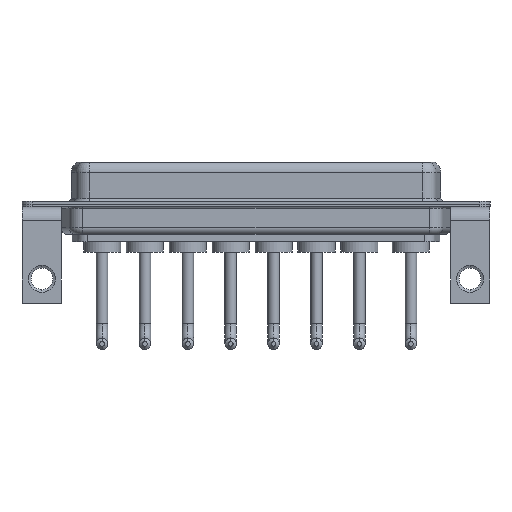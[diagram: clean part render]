
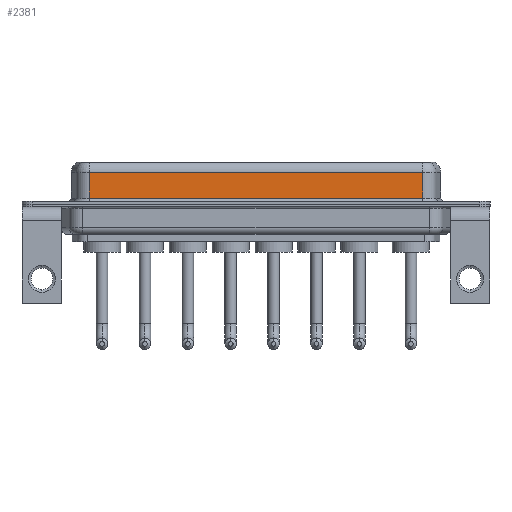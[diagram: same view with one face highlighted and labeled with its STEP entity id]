
A CAD part, front view. The second image highlights one B-rep face of the part: STEP entity #2381.
In plain terms, the highlighted planar face has unit normal (0, -1, 0).
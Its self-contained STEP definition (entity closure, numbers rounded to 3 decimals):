
#185 = VERTEX_POINT ( 'NONE', #13521 ) ;
#1235 = CARTESIAN_POINT ( 'NONE',  ( 56.462, -3.95, 0.9 ) ) ;
#1314 = CARTESIAN_POINT ( 'NONE',  ( 56.462, -3.95, 0.9 ) ) ;
#1459 = ORIENTED_EDGE ( 'NONE', *, *, #13562, .T. ) ;
#1554 = CARTESIAN_POINT ( 'NONE',  ( 7.038, -3.95, 0.9 ) ) ;
#1815 = DIRECTION ( 'NONE',  ( -1., 0., 0. ) ) ;
#2146 = VECTOR ( 'NONE', #1815, 1000. ) ;
#2158 = DIRECTION ( 'NONE',  ( 1., 0., 0. ) ) ;
#2282 = CARTESIAN_POINT ( 'NONE',  ( 56.462, -3.95, 4.65 ) ) ;
#2297 = VECTOR ( 'NONE', #3578, 1000. ) ;
#2381 = ADVANCED_FACE ( 'NONE', ( #13694 ), #3968, .F. ) ;
#2827 = DIRECTION ( 'NONE',  ( 0., 1., 0. ) ) ;
#3151 = EDGE_CURVE ( 'NONE', #6410, #12816, #8992, .T. ) ;
#3353 = CARTESIAN_POINT ( 'NONE',  ( 7.038, -3.95, 4.65 ) ) ;
#3578 = DIRECTION ( 'NONE',  ( 0., 0., -1. ) ) ;
#3968 = PLANE ( 'NONE',  #8597 ) ;
#3984 = EDGE_CURVE ( 'NONE', #13547, #6410, #8546, .T. ) ;
#4740 = DIRECTION ( 'NONE',  ( 0., 0., -1. ) ) ;
#4902 = DIRECTION ( 'NONE',  ( 0., 0., 1. ) ) ;
#5566 = VECTOR ( 'NONE', #4740, 1000. ) ;
#5620 = EDGE_LOOP ( 'NONE', ( #9661, #1459, #6217, #13691 ) ) ;
#6217 = ORIENTED_EDGE ( 'NONE', *, *, #3984, .T. ) ;
#6410 = VERTEX_POINT ( 'NONE', #1554 ) ;
#6791 = LINE ( 'NONE', #10136, #5566 ) ;
#7906 = EDGE_CURVE ( 'NONE', #185, #12816, #6791, .T. ) ;
#8213 = CARTESIAN_POINT ( 'NONE',  ( 56.462, -3.95, 6.4 ) ) ;
#8546 = LINE ( 'NONE', #9109, #2297 ) ;
#8597 = AXIS2_PLACEMENT_3D ( 'NONE', #8213, #2827, #4902 ) ;
#8992 = LINE ( 'NONE', #1235, #11209 ) ;
#9109 = CARTESIAN_POINT ( 'NONE',  ( 7.038, -3.95, 6.4 ) ) ;
#9661 = ORIENTED_EDGE ( 'NONE', *, *, #7906, .F. ) ;
#10136 = CARTESIAN_POINT ( 'NONE',  ( 56.462, -3.95, 6.4 ) ) ;
#11209 = VECTOR ( 'NONE', #2158, 1000. ) ;
#12034 = LINE ( 'NONE', #2282, #2146 ) ;
#12816 = VERTEX_POINT ( 'NONE', #1314 ) ;
#13521 = CARTESIAN_POINT ( 'NONE',  ( 56.462, -3.95, 4.65 ) ) ;
#13547 = VERTEX_POINT ( 'NONE', #3353 ) ;
#13562 = EDGE_CURVE ( 'NONE', #185, #13547, #12034, .T. ) ;
#13691 = ORIENTED_EDGE ( 'NONE', *, *, #3151, .T. ) ;
#13694 = FACE_OUTER_BOUND ( 'NONE', #5620, .T. ) ;
